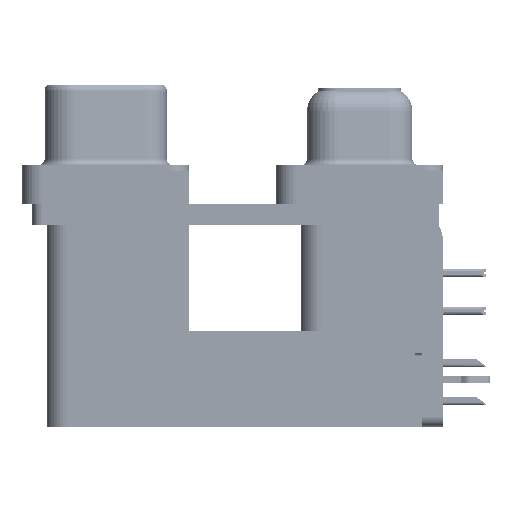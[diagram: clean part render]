
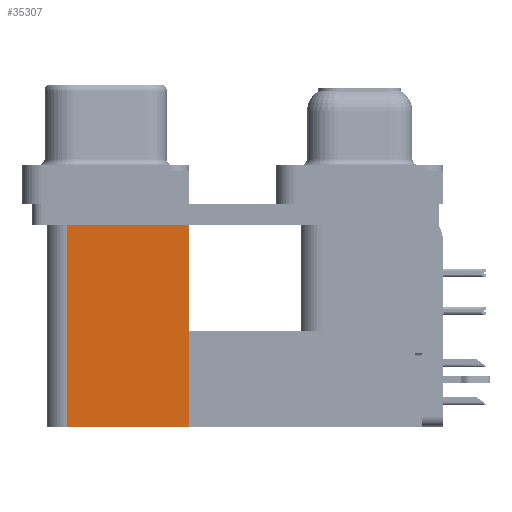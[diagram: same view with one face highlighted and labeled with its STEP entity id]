
A CAD part, left-side view. The second image highlights one B-rep face of the part: STEP entity #35307.
In plain terms, the highlighted planar face has unit normal (-1, 0, 0).
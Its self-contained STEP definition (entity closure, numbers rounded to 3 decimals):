
#1399 = EDGE_CURVE ( 'NONE', #36246, #18020, #47748, .T. ) ;
#6924 = DIRECTION ( 'NONE',  ( 0., 1., 0. ) ) ;
#8671 = LINE ( 'NONE', #9648, #51438 ) ;
#9648 = CARTESIAN_POINT ( 'NONE',  ( 3.79, 12.775, -19.2 ) ) ;
#10387 = LINE ( 'NONE', #30823, #17622 ) ;
#10727 = LINE ( 'NONE', #14503, #64244 ) ;
#13083 = ORIENTED_EDGE ( 'NONE', *, *, #1399, .T. ) ;
#14503 = CARTESIAN_POINT ( 'NONE',  ( 3.79, 21.975, -19.2 ) ) ;
#17622 = VECTOR ( 'NONE', #62395, 1000. ) ;
#18020 = VERTEX_POINT ( 'NONE', #54638 ) ;
#18466 = FACE_OUTER_BOUND ( 'NONE', #55344, .T. ) ;
#20537 = CARTESIAN_POINT ( 'NONE',  ( 3.79, 21.975, -19.2 ) ) ;
#20916 = CARTESIAN_POINT ( 'NONE',  ( 3.79, 12.775, -2.5 ) ) ;
#25349 = CARTESIAN_POINT ( 'NONE',  ( 3.79, 12.775, -2.5 ) ) ;
#27256 = ORIENTED_EDGE ( 'NONE', *, *, #29097, .T. ) ;
#29092 = EDGE_CURVE ( 'NONE', #43416, #18020, #10727, .T. ) ;
#29097 = EDGE_CURVE ( 'NONE', #42748, #36246, #10387, .T. ) ;
#30823 = CARTESIAN_POINT ( 'NONE',  ( 3.79, 12.775, -19.2 ) ) ;
#32582 = ORIENTED_EDGE ( 'NONE', *, *, #29092, .F. ) ;
#32773 = DIRECTION ( 'NONE',  ( 1., 0., 0. ) ) ;
#32945 = EDGE_CURVE ( 'NONE', #42748, #43416, #8671, .T. ) ;
#35307 = ADVANCED_FACE ( 'NONE', ( #18466 ), #63676, .F. ) ;
#36246 = VERTEX_POINT ( 'NONE', #25349 ) ;
#36893 = DIRECTION ( 'NONE',  ( 0., 1., 0. ) ) ;
#37704 = VECTOR ( 'NONE', #36893, 1000. ) ;
#37959 = AXIS2_PLACEMENT_3D ( 'NONE', #49050, #32773, #6924 ) ;
#40823 = ORIENTED_EDGE ( 'NONE', *, *, #32945, .F. ) ;
#42748 = VERTEX_POINT ( 'NONE', #44457 ) ;
#43416 = VERTEX_POINT ( 'NONE', #20537 ) ;
#44457 = CARTESIAN_POINT ( 'NONE',  ( 3.79, 12.775, -19.2 ) ) ;
#45368 = DIRECTION ( 'NONE',  ( 0., 1., 0. ) ) ;
#46431 = DIRECTION ( 'NONE',  ( 0., 0., 1. ) ) ;
#47748 = LINE ( 'NONE', #20916, #37704 ) ;
#49050 = CARTESIAN_POINT ( 'NONE',  ( 3.79, 12.775, -19.2 ) ) ;
#51438 = VECTOR ( 'NONE', #45368, 1000. ) ;
#54638 = CARTESIAN_POINT ( 'NONE',  ( 3.79, 21.975, -2.5 ) ) ;
#55344 = EDGE_LOOP ( 'NONE', ( #13083, #32582, #40823, #27256 ) ) ;
#62395 = DIRECTION ( 'NONE',  ( 0., 0., 1. ) ) ;
#63676 = PLANE ( 'NONE',  #37959 ) ;
#64244 = VECTOR ( 'NONE', #46431, 1000. ) ;
